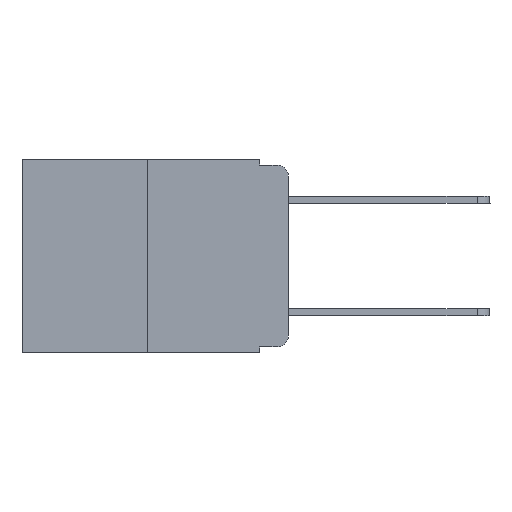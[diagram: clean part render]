
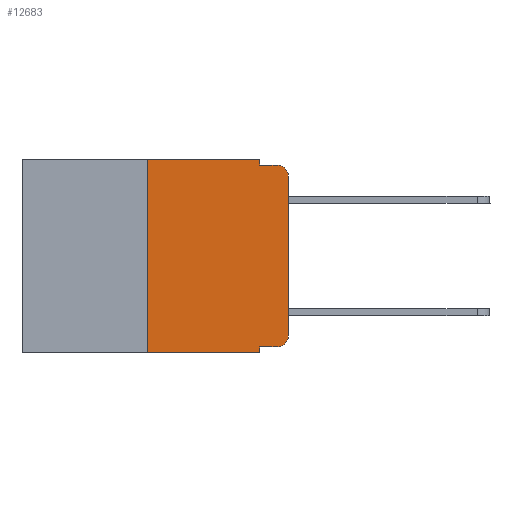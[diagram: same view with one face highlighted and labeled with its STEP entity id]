
A CAD part, left-side view. The second image highlights one B-rep face of the part: STEP entity #12683.
In plain terms, the highlighted planar face has unit normal (-1, 0, 0).
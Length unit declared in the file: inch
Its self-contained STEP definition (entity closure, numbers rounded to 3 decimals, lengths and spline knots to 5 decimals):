
#27 = DIRECTION ( 'NONE',  ( 0., 0., -1. ) ) ;
#153 = ORIENTED_EDGE ( 'NONE', *, *, #9383, .F. ) ;
#160 = EDGE_CURVE ( 'NONE', #4053, #1095, #7732, .T. ) ;
#504 = CARTESIAN_POINT ( 'NONE',  ( 0., 0.02, -0.01 ) ) ;
#615 = CARTESIAN_POINT ( 'NONE',  ( 0., 0.473, 0. ) ) ;
#717 = LINE ( 'NONE', #11826, #3566 ) ;
#747 = VERTEX_POINT ( 'NONE', #8539 ) ;
#792 = CARTESIAN_POINT ( 'NONE',  ( 0., 0.02, -0.03 ) ) ;
#822 = CIRCLE ( 'NONE', #11376, 0.02 ) ;
#887 = ORIENTED_EDGE ( 'NONE', *, *, #1966, .F. ) ;
#1050 = AXIS2_PLACEMENT_3D ( 'NONE', #615, #7384, #5136 ) ;
#1095 = VERTEX_POINT ( 'NONE', #7820 ) ;
#1134 = VERTEX_POINT ( 'NONE', #3107 ) ;
#1193 = VERTEX_POINT ( 'NONE', #7720 ) ;
#1398 = ORIENTED_EDGE ( 'NONE', *, *, #10657, .T. ) ;
#1451 = FACE_OUTER_BOUND ( 'NONE', #9324, .T. ) ;
#1516 = CARTESIAN_POINT ( 'NONE',  ( 0., 0.25, 0. ) ) ;
#1612 = VECTOR ( 'NONE', #4034, 39.37008 ) ;
#1615 = DIRECTION ( 'NONE',  ( 0., 0., 1. ) ) ;
#1640 = PLANE ( 'NONE',  #1050 ) ;
#1663 = VECTOR ( 'NONE', #2117, 39.37008 ) ;
#1692 = ORIENTED_EDGE ( 'NONE', *, *, #160, .T. ) ;
#1694 = VECTOR ( 'NONE', #5484, 39.37008 ) ;
#1966 = EDGE_CURVE ( 'NONE', #1193, #11546, #5259, .T. ) ;
#2117 = DIRECTION ( 'NONE',  ( 0., -1., 0. ) ) ;
#2188 = CARTESIAN_POINT ( 'NONE',  ( 0., 0.473, 0. ) ) ;
#2267 = VECTOR ( 'NONE', #1615, 39.37008 ) ;
#2583 = LINE ( 'NONE', #10373, #2267 ) ;
#2648 = DIRECTION ( 'NONE',  ( 0., 0., -1. ) ) ;
#3107 = CARTESIAN_POINT ( 'NONE',  ( 0., 0.25, -0.343 ) ) ;
#3480 = CIRCLE ( 'NONE', #3897, 0.02 ) ;
#3526 = VERTEX_POINT ( 'NONE', #5025 ) ;
#3566 = VECTOR ( 'NONE', #7690, 39.37008 ) ;
#3578 = DIRECTION ( 'NONE',  ( 0., -1., 0. ) ) ;
#3592 = LINE ( 'NONE', #9721, #5595 ) ;
#3897 = AXIS2_PLACEMENT_3D ( 'NONE', #792, #7492, #2648 ) ;
#4034 = DIRECTION ( 'NONE',  ( 0., -1., 0. ) ) ;
#4053 = VERTEX_POINT ( 'NONE', #5010 ) ;
#4266 = VERTEX_POINT ( 'NONE', #7453 ) ;
#4804 = CARTESIAN_POINT ( 'NONE',  ( 0., 0.473, -0.343 ) ) ;
#5010 = CARTESIAN_POINT ( 'NONE',  ( 0., 0.051, -0.333 ) ) ;
#5025 = CARTESIAN_POINT ( 'NONE',  ( 0., 0., -0.313 ) ) ;
#5136 = DIRECTION ( 'NONE',  ( 0., 0., -1. ) ) ;
#5171 = CARTESIAN_POINT ( 'NONE',  ( 0., 0.051, -0.01 ) ) ;
#5259 = LINE ( 'NONE', #9056, #5874 ) ;
#5484 = DIRECTION ( 'NONE',  ( 0., -1., 0. ) ) ;
#5595 = VECTOR ( 'NONE', #9582, 39.37008 ) ;
#5874 = VECTOR ( 'NONE', #7089, 39.37008 ) ;
#6767 = ORIENTED_EDGE ( 'NONE', *, *, #10635, .T. ) ;
#7089 = DIRECTION ( 'NONE',  ( 0., 0., -1. ) ) ;
#7192 = LINE ( 'NONE', #10998, #1663 ) ;
#7384 = DIRECTION ( 'NONE',  ( 1., 0., 0. ) ) ;
#7453 = CARTESIAN_POINT ( 'NONE',  ( 0., 0.051, -0.343 ) ) ;
#7492 = DIRECTION ( 'NONE',  ( -1., 0., 0. ) ) ;
#7555 = EDGE_CURVE ( 'NONE', #4053, #4266, #3592, .T. ) ;
#7572 = EDGE_CURVE ( 'NONE', #1134, #8311, #717, .T. ) ;
#7602 = LINE ( 'NONE', #4804, #8023 ) ;
#7654 = ORIENTED_EDGE ( 'NONE', *, *, #10326, .T. ) ;
#7690 = DIRECTION ( 'NONE',  ( 0., 0., 1. ) ) ;
#7720 = CARTESIAN_POINT ( 'NONE',  ( 0., 0.051, 0. ) ) ;
#7732 = LINE ( 'NONE', #8853, #1694 ) ;
#7820 = CARTESIAN_POINT ( 'NONE',  ( 0., 0.02, -0.333 ) ) ;
#7918 = ORIENTED_EDGE ( 'NONE', *, *, #9240, .T. ) ;
#8023 = VECTOR ( 'NONE', #3578, 39.37008 ) ;
#8311 = VERTEX_POINT ( 'NONE', #1516 ) ;
#8539 = CARTESIAN_POINT ( 'NONE',  ( 0., 0., -0.03 ) ) ;
#8850 = ORIENTED_EDGE ( 'NONE', *, *, #7572, .F. ) ;
#8853 = CARTESIAN_POINT ( 'NONE',  ( 0., 0.051, -0.333 ) ) ;
#9056 = CARTESIAN_POINT ( 'NONE',  ( 0., 0.051, 0. ) ) ;
#9093 = VERTEX_POINT ( 'NONE', #504 ) ;
#9240 = EDGE_CURVE ( 'NONE', #1134, #4266, #7602, .T. ) ;
#9324 = EDGE_LOOP ( 'NONE', ( #1398, #6767, #12293, #887, #153, #8850, #7918, #12173, #1692, #7654 ) ) ;
#9383 = EDGE_CURVE ( 'NONE', #8311, #1193, #9972, .T. ) ;
#9582 = DIRECTION ( 'NONE',  ( 0., 0., -1. ) ) ;
#9721 = CARTESIAN_POINT ( 'NONE',  ( 0., 0.051, 0. ) ) ;
#9872 = DIRECTION ( 'NONE',  ( -1., 0., 0. ) ) ;
#9972 = LINE ( 'NONE', #2188, #1612 ) ;
#10003 = CARTESIAN_POINT ( 'NONE',  ( 0., 0.02, -0.313 ) ) ;
#10326 = EDGE_CURVE ( 'NONE', #1095, #3526, #822, .T. ) ;
#10373 = CARTESIAN_POINT ( 'NONE',  ( 0., 0., 0. ) ) ;
#10635 = EDGE_CURVE ( 'NONE', #747, #9093, #3480, .T. ) ;
#10657 = EDGE_CURVE ( 'NONE', #3526, #747, #2583, .T. ) ;
#10998 = CARTESIAN_POINT ( 'NONE',  ( 0., 0.051, -0.01 ) ) ;
#11259 = EDGE_CURVE ( 'NONE', #11546, #9093, #7192, .T. ) ;
#11376 = AXIS2_PLACEMENT_3D ( 'NONE', #10003, #9872, #27 ) ;
#11546 = VERTEX_POINT ( 'NONE', #5171 ) ;
#11826 = CARTESIAN_POINT ( 'NONE',  ( 0., 0.25, 0. ) ) ;
#12173 = ORIENTED_EDGE ( 'NONE', *, *, #7555, .F. ) ;
#12293 = ORIENTED_EDGE ( 'NONE', *, *, #11259, .F. ) ;
#12683 = ADVANCED_FACE ( 'NONE', ( #1451 ), #1640, .F. ) ;
